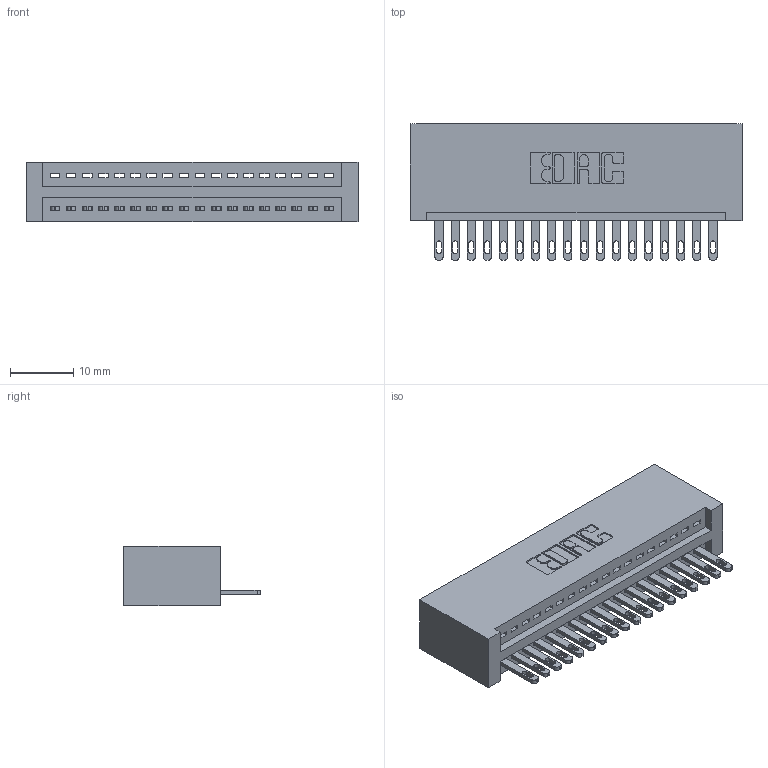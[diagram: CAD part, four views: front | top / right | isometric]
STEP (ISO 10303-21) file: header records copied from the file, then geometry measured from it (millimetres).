
FILE_DESCRIPTION (( 'STEP AP203' ), '1' );
FILE_NAME ('345-018-500-101.STEP', '2019-10-04T16:35:21', ( '' ), ( '' ), 'SwSTEP 2.0', 'SolidWorks 2016', '' );
FILE_SCHEMA (( 'CONFIG_CONTROL_DESIGN' ));
Length unit declared in the file: inch
Products named in the file (3): 345-292-001_345-293-100; 345-018-500-101; 345 Part_No Mounting Lugs
Assembly tree (19 placements, depth 2):
  345-018-500-101
    345 Part_No Mounting Lugs
    345-292-001_345-293-100  x18
Bounding box: 52.32 x 21.51 x 9.4 mm (x, y, z)
Volume: 5368.7 mm3; surface area: 7038.9 mm2
Topology: 19 solids, 19 shells, 1090 faces, 3341 edges, 2226 vertices
Faces by surface type: plane 688, cylinder 402
Entity records: 16431 total; most frequent: CARTESIAN_POINT 2854, ORIENTED_EDGE 2806, DIRECTION 2523, EDGE_CURVE 1403, LINE 1203, VECTOR 1203, VERTEX_POINT 934, AXIS2_PLACEMENT_3D 660
